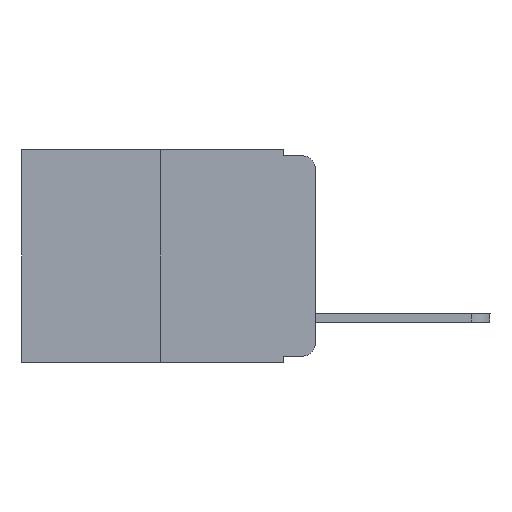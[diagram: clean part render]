
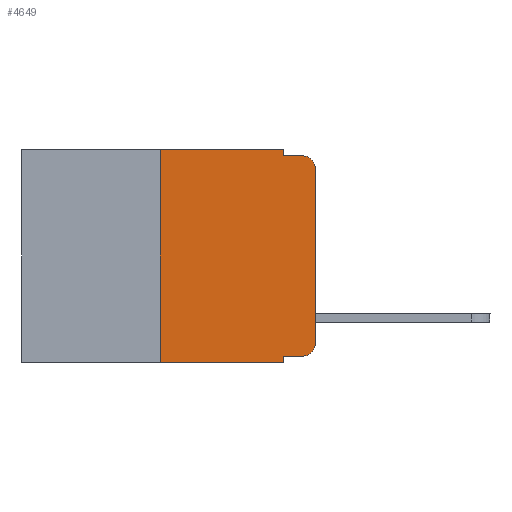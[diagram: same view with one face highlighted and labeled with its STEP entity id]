
A CAD part, left-side view. The second image highlights one B-rep face of the part: STEP entity #4649.
In plain terms, the highlighted planar face has unit normal (-1, 0, 0).
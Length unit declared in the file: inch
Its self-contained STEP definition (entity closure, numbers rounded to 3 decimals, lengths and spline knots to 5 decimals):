
#364 = EDGE_CURVE ( 'NONE', #11366, #19734, #20401, .T. ) ;
#569 = ORIENTED_EDGE ( 'NONE', *, *, #19128, .T. ) ;
#825 = VECTOR ( 'NONE', #1900, 39.37008 ) ;
#1053 = LINE ( 'NONE', #19671, #3350 ) ;
#1213 = EDGE_CURVE ( 'NONE', #4719, #15693, #1053, .T. ) ;
#1553 = VERTEX_POINT ( 'NONE', #2419 ) ;
#1630 = EDGE_LOOP ( 'NONE', ( #9665, #22539, #1915, #10556, #20158, #1849, #6901, #7218, #21697, #569 ) ) ;
#1849 = ORIENTED_EDGE ( 'NONE', *, *, #5550, .F. ) ;
#1889 = LINE ( 'NONE', #12283, #18617 ) ;
#1900 = DIRECTION ( 'NONE',  ( 0., -1., 0. ) ) ;
#1915 = ORIENTED_EDGE ( 'NONE', *, *, #18214, .F. ) ;
#1979 = EDGE_CURVE ( 'NONE', #15693, #6906, #22579, .T. ) ;
#2419 = CARTESIAN_POINT ( 'NONE',  ( 0., 0.02, -0.333 ) ) ;
#2562 = VECTOR ( 'NONE', #18151, 39.37008 ) ;
#2647 = CARTESIAN_POINT ( 'NONE',  ( 0., 0.051, 0. ) ) ;
#3350 = VECTOR ( 'NONE', #14182, 39.37008 ) ;
#3408 = VERTEX_POINT ( 'NONE', #16706 ) ;
#4028 = VERTEX_POINT ( 'NONE', #4444 ) ;
#4413 = PLANE ( 'NONE',  #17822 ) ;
#4444 = CARTESIAN_POINT ( 'NONE',  ( 0., 0., -0.313 ) ) ;
#4649 = ADVANCED_FACE ( 'NONE', ( #5866 ), #4413, .F. ) ;
#4719 = VERTEX_POINT ( 'NONE', #6666 ) ;
#5526 = VECTOR ( 'NONE', #16848, 39.37008 ) ;
#5545 = EDGE_CURVE ( 'NONE', #4028, #11955, #1889, .T. ) ;
#5550 = EDGE_CURVE ( 'NONE', #11366, #4719, #22038, .T. ) ;
#5644 = CARTESIAN_POINT ( 'NONE',  ( 0., 0.02, -0.01 ) ) ;
#5766 = CARTESIAN_POINT ( 'NONE',  ( 0., 0.051, -0.343 ) ) ;
#5866 = FACE_OUTER_BOUND ( 'NONE', #1630, .T. ) ;
#5915 = CIRCLE ( 'NONE', #11673, 0.02 ) ;
#5992 = CARTESIAN_POINT ( 'NONE',  ( 0., 0., -0.03 ) ) ;
#6111 = DIRECTION ( 'NONE',  ( 0., 0., -1. ) ) ;
#6487 = LINE ( 'NONE', #19822, #2562 ) ;
#6583 = DIRECTION ( 'NONE',  ( 0., 0., -1. ) ) ;
#6617 = VECTOR ( 'NONE', #12783, 39.37008 ) ;
#6666 = CARTESIAN_POINT ( 'NONE',  ( 0., 0.25, 0. ) ) ;
#6901 = ORIENTED_EDGE ( 'NONE', *, *, #364, .T. ) ;
#6906 = VERTEX_POINT ( 'NONE', #11775 ) ;
#7218 = ORIENTED_EDGE ( 'NONE', *, *, #13702, .F. ) ;
#8046 = CARTESIAN_POINT ( 'NONE',  ( 0., 0.473, 0. ) ) ;
#9601 = CARTESIAN_POINT ( 'NONE',  ( 0., 0.051, -0.01 ) ) ;
#9665 = ORIENTED_EDGE ( 'NONE', *, *, #5545, .T. ) ;
#9786 = DIRECTION ( 'NONE',  ( -1., 0., 0. ) ) ;
#9849 = EDGE_CURVE ( 'NONE', #3408, #1553, #6487, .T. ) ;
#9855 = EDGE_CURVE ( 'NONE', #11955, #16953, #5915, .T. ) ;
#10140 = CARTESIAN_POINT ( 'NONE',  ( 0., 0.25, -0.343 ) ) ;
#10556 = ORIENTED_EDGE ( 'NONE', *, *, #1979, .F. ) ;
#10822 = CARTESIAN_POINT ( 'NONE',  ( 0., 0.051, 0. ) ) ;
#11366 = VERTEX_POINT ( 'NONE', #10140 ) ;
#11673 = AXIS2_PLACEMENT_3D ( 'NONE', #21711, #18224, #12679 ) ;
#11775 = CARTESIAN_POINT ( 'NONE',  ( 0., 0.051, -0.01 ) ) ;
#11955 = VERTEX_POINT ( 'NONE', #5992 ) ;
#12283 = CARTESIAN_POINT ( 'NONE',  ( 0., 0., 0. ) ) ;
#12679 = DIRECTION ( 'NONE',  ( 0., 0., -1. ) ) ;
#12783 = DIRECTION ( 'NONE',  ( 0., 0., -1. ) ) ;
#13603 = VECTOR ( 'NONE', #22279, 39.37008 ) ;
#13702 = EDGE_CURVE ( 'NONE', #3408, #19734, #18850, .T. ) ;
#14182 = DIRECTION ( 'NONE',  ( 0., -1., 0. ) ) ;
#14261 = DIRECTION ( 'NONE',  ( 0., 0., 1. ) ) ;
#15001 = AXIS2_PLACEMENT_3D ( 'NONE', #15404, #9786, #6111 ) ;
#15404 = CARTESIAN_POINT ( 'NONE',  ( 0., 0.02, -0.313 ) ) ;
#15693 = VERTEX_POINT ( 'NONE', #16854 ) ;
#16082 = VECTOR ( 'NONE', #23291, 39.37008 ) ;
#16706 = CARTESIAN_POINT ( 'NONE',  ( 0., 0.051, -0.333 ) ) ;
#16848 = DIRECTION ( 'NONE',  ( 0., 0., -1. ) ) ;
#16854 = CARTESIAN_POINT ( 'NONE',  ( 0., 0.051, 0. ) ) ;
#16953 = VERTEX_POINT ( 'NONE', #5644 ) ;
#17540 = CIRCLE ( 'NONE', #15001, 0.02 ) ;
#17822 = AXIS2_PLACEMENT_3D ( 'NONE', #8046, #20748, #6583 ) ;
#18151 = DIRECTION ( 'NONE',  ( 0., -1., 0. ) ) ;
#18214 = EDGE_CURVE ( 'NONE', #6906, #16953, #22388, .T. ) ;
#18224 = DIRECTION ( 'NONE',  ( -1., 0., 0. ) ) ;
#18617 = VECTOR ( 'NONE', #14261, 39.37008 ) ;
#18850 = LINE ( 'NONE', #10822, #6617 ) ;
#19128 = EDGE_CURVE ( 'NONE', #1553, #4028, #17540, .T. ) ;
#19671 = CARTESIAN_POINT ( 'NONE',  ( 0., 0.473, 0. ) ) ;
#19734 = VERTEX_POINT ( 'NONE', #5766 ) ;
#19822 = CARTESIAN_POINT ( 'NONE',  ( 0., 0.051, -0.333 ) ) ;
#20158 = ORIENTED_EDGE ( 'NONE', *, *, #1213, .F. ) ;
#20401 = LINE ( 'NONE', #21542, #825 ) ;
#20748 = DIRECTION ( 'NONE',  ( 1., 0., 0. ) ) ;
#21477 = CARTESIAN_POINT ( 'NONE',  ( 0., 0.25, 0. ) ) ;
#21542 = CARTESIAN_POINT ( 'NONE',  ( 0., 0.473, -0.343 ) ) ;
#21697 = ORIENTED_EDGE ( 'NONE', *, *, #9849, .T. ) ;
#21711 = CARTESIAN_POINT ( 'NONE',  ( 0., 0.02, -0.03 ) ) ;
#22038 = LINE ( 'NONE', #21477, #16082 ) ;
#22279 = DIRECTION ( 'NONE',  ( 0., -1., 0. ) ) ;
#22388 = LINE ( 'NONE', #9601, #13603 ) ;
#22539 = ORIENTED_EDGE ( 'NONE', *, *, #9855, .T. ) ;
#22579 = LINE ( 'NONE', #2647, #5526 ) ;
#23291 = DIRECTION ( 'NONE',  ( 0., 0., 1. ) ) ;
